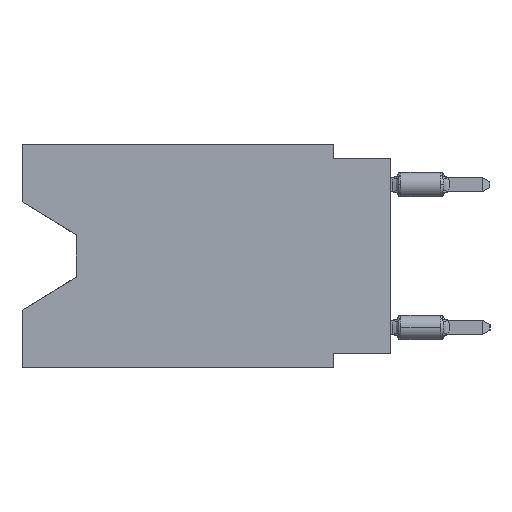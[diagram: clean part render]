
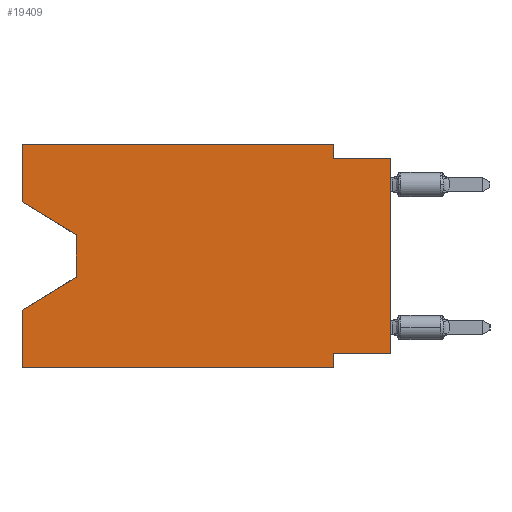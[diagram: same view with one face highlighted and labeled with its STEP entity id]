
A CAD part, left-side view. The second image highlights one B-rep face of the part: STEP entity #19409.
In plain terms, the highlighted planar face has unit normal (-1, 0, 0).
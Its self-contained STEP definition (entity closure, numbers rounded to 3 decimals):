
#769 = LINE ( 'NONE', #37833, #2284 ) ;
#1175 = EDGE_CURVE ( 'NONE', #31974, #5391, #14698, .T. ) ;
#2036 = VERTEX_POINT ( 'NONE', #26834 ) ;
#2257 = EDGE_CURVE ( 'NONE', #15369, #25158, #39160, .T. ) ;
#2284 = VECTOR ( 'NONE', #16384, 1000. ) ;
#2491 = ORIENTED_EDGE ( 'NONE', *, *, #31625, .F. ) ;
#2535 = ORIENTED_EDGE ( 'NONE', *, *, #34616, .T. ) ;
#2541 = LINE ( 'NONE', #26985, #7449 ) ;
#3087 = DIRECTION ( 'NONE',  ( 0., 0., -1. ) ) ;
#3684 = VECTOR ( 'NONE', #36802, 1000. ) ;
#3705 = VECTOR ( 'NONE', #6107, 1000. ) ;
#4490 = VERTEX_POINT ( 'NONE', #18574 ) ;
#4748 = VERTEX_POINT ( 'NONE', #14149 ) ;
#5391 = VERTEX_POINT ( 'NONE', #8476 ) ;
#5702 = EDGE_CURVE ( 'NONE', #15369, #31974, #36224, .T. ) ;
#5930 = ORIENTED_EDGE ( 'NONE', *, *, #35896, .F. ) ;
#6107 = DIRECTION ( 'NONE',  ( 0., -1., 0. ) ) ;
#6384 = EDGE_LOOP ( 'NONE', ( #8513, #2535, #28436, #39403, #6542, #34050, #6508, #29250, #2491, #23176, #24631, #5930 ) ) ;
#6508 = ORIENTED_EDGE ( 'NONE', *, *, #5702, .F. ) ;
#6542 = ORIENTED_EDGE ( 'NONE', *, *, #36225, .T. ) ;
#6558 = CARTESIAN_POINT ( 'NONE',  ( 0., 16.383, 0. ) ) ;
#6977 = LINE ( 'NONE', #6558, #18421 ) ;
#7378 = DIRECTION ( 'NONE',  ( 0., -0.855, -0.519 ) ) ;
#7383 = CARTESIAN_POINT ( 'NONE',  ( 0., 13.97, -4.013 ) ) ;
#7449 = VECTOR ( 'NONE', #32606, 1000. ) ;
#8476 = CARTESIAN_POINT ( 'NONE',  ( 0., 2.54, -9.906 ) ) ;
#8513 = ORIENTED_EDGE ( 'NONE', *, *, #14621, .T. ) ;
#9091 = CARTESIAN_POINT ( 'NONE',  ( 0., 2.54, 0. ) ) ;
#9476 = VERTEX_POINT ( 'NONE', #14337 ) ;
#11673 = DIRECTION ( 'NONE',  ( 0., 0., -1. ) ) ;
#11680 = DIRECTION ( 'NONE',  ( 0., 0., 1. ) ) ;
#12009 = VERTEX_POINT ( 'NONE', #27148 ) ;
#12257 = VERTEX_POINT ( 'NONE', #38167 ) ;
#12386 = AXIS2_PLACEMENT_3D ( 'NONE', #30185, #30781, #15367 ) ;
#13312 = CARTESIAN_POINT ( 'NONE',  ( 0., 2.54, -9.271 ) ) ;
#13584 = VECTOR ( 'NONE', #11673, 1000. ) ;
#14046 = CARTESIAN_POINT ( 'NONE',  ( 0., 0., -0.635 ) ) ;
#14149 = CARTESIAN_POINT ( 'NONE',  ( 0., 2.54, 0. ) ) ;
#14337 = CARTESIAN_POINT ( 'NONE',  ( 0., 13.97, -4.013 ) ) ;
#14621 = EDGE_CURVE ( 'NONE', #4490, #9476, #22603, .T. ) ;
#14698 = LINE ( 'NONE', #39154, #13584 ) ;
#15223 = VECTOR ( 'NONE', #35981, 1000. ) ;
#15367 = DIRECTION ( 'NONE',  ( 0., 0., -1. ) ) ;
#15369 = VERTEX_POINT ( 'NONE', #19131 ) ;
#15657 = VECTOR ( 'NONE', #7378, 1000. ) ;
#15848 = EDGE_CURVE ( 'NONE', #12257, #2036, #20581, .T. ) ;
#16024 = DIRECTION ( 'NONE',  ( 0., 0., -1. ) ) ;
#16384 = DIRECTION ( 'NONE',  ( 0., -1., 0. ) ) ;
#18382 = CARTESIAN_POINT ( 'NONE',  ( 0., 0., -9.271 ) ) ;
#18421 = VECTOR ( 'NONE', #37226, 1000. ) ;
#18574 = CARTESIAN_POINT ( 'NONE',  ( 0., 16.383, -2.546 ) ) ;
#19131 = CARTESIAN_POINT ( 'NONE',  ( 0., 0., -9.271 ) ) ;
#19409 = ADVANCED_FACE ( 'NONE', ( #36782 ), #24192, .F. ) ;
#20394 = DIRECTION ( 'NONE',  ( 0., 0., 1. ) ) ;
#20454 = CARTESIAN_POINT ( 'NONE',  ( 0., 2.54, -0.635 ) ) ;
#20505 = CARTESIAN_POINT ( 'NONE',  ( 0., 0., 0. ) ) ;
#20550 = LINE ( 'NONE', #32773, #3705 ) ;
#20581 = LINE ( 'NONE', #38463, #32986 ) ;
#22603 = LINE ( 'NONE', #34820, #15657 ) ;
#23176 = ORIENTED_EDGE ( 'NONE', *, *, #32503, .F. ) ;
#23761 = LINE ( 'NONE', #29973, #15223 ) ;
#24192 = PLANE ( 'NONE',  #12386 ) ;
#24631 = ORIENTED_EDGE ( 'NONE', *, *, #36163, .F. ) ;
#24633 = CARTESIAN_POINT ( 'NONE',  ( 0., 13.97, -5.893 ) ) ;
#25158 = VERTEX_POINT ( 'NONE', #14046 ) ;
#26140 = VECTOR ( 'NONE', #16024, 1000. ) ;
#26834 = CARTESIAN_POINT ( 'NONE',  ( 0., 16.383, -7.36 ) ) ;
#26985 = CARTESIAN_POINT ( 'NONE',  ( 0., 13.97, -5.893 ) ) ;
#27148 = CARTESIAN_POINT ( 'NONE',  ( 0., 16.383, 0. ) ) ;
#27702 = VECTOR ( 'NONE', #11680, 1000. ) ;
#27922 = LINE ( 'NONE', #9091, #34968 ) ;
#28436 = ORIENTED_EDGE ( 'NONE', *, *, #39083, .T. ) ;
#28625 = VERTEX_POINT ( 'NONE', #24633 ) ;
#29250 = ORIENTED_EDGE ( 'NONE', *, *, #2257, .T. ) ;
#29973 = CARTESIAN_POINT ( 'NONE',  ( 0., 16.383, -9.906 ) ) ;
#30185 = CARTESIAN_POINT ( 'NONE',  ( 0., 16.383, 0. ) ) ;
#30781 = DIRECTION ( 'NONE',  ( 1., 0., 0. ) ) ;
#31625 = EDGE_CURVE ( 'NONE', #35537, #25158, #769, .T. ) ;
#31974 = VERTEX_POINT ( 'NONE', #13312 ) ;
#32503 = EDGE_CURVE ( 'NONE', #4748, #35537, #27922, .T. ) ;
#32606 = DIRECTION ( 'NONE',  ( 0., 0.855, -0.519 ) ) ;
#32773 = CARTESIAN_POINT ( 'NONE',  ( 0., 16.383, 0. ) ) ;
#32986 = VECTOR ( 'NONE', #20394, 1000. ) ;
#34050 = ORIENTED_EDGE ( 'NONE', *, *, #1175, .F. ) ;
#34616 = EDGE_CURVE ( 'NONE', #9476, #28625, #34825, .T. ) ;
#34820 = CARTESIAN_POINT ( 'NONE',  ( 0., 16.383, -2.546 ) ) ;
#34825 = LINE ( 'NONE', #7383, #26140 ) ;
#34968 = VECTOR ( 'NONE', #3087, 1000. ) ;
#35537 = VERTEX_POINT ( 'NONE', #20454 ) ;
#35896 = EDGE_CURVE ( 'NONE', #4490, #12009, #6977, .T. ) ;
#35981 = DIRECTION ( 'NONE',  ( 0., -1., 0. ) ) ;
#36163 = EDGE_CURVE ( 'NONE', #12009, #4748, #20550, .T. ) ;
#36224 = LINE ( 'NONE', #18382, #3684 ) ;
#36225 = EDGE_CURVE ( 'NONE', #12257, #5391, #23761, .T. ) ;
#36782 = FACE_OUTER_BOUND ( 'NONE', #6384, .T. ) ;
#36802 = DIRECTION ( 'NONE',  ( 0., 1., 0. ) ) ;
#37226 = DIRECTION ( 'NONE',  ( 0., 0., 1. ) ) ;
#37833 = CARTESIAN_POINT ( 'NONE',  ( 0., 0., -0.635 ) ) ;
#38167 = CARTESIAN_POINT ( 'NONE',  ( 0., 16.383, -9.906 ) ) ;
#38463 = CARTESIAN_POINT ( 'NONE',  ( 0., 16.383, 0. ) ) ;
#39083 = EDGE_CURVE ( 'NONE', #28625, #2036, #2541, .T. ) ;
#39154 = CARTESIAN_POINT ( 'NONE',  ( 0., 2.54, -9.906 ) ) ;
#39160 = LINE ( 'NONE', #20505, #27702 ) ;
#39403 = ORIENTED_EDGE ( 'NONE', *, *, #15848, .F. ) ;
